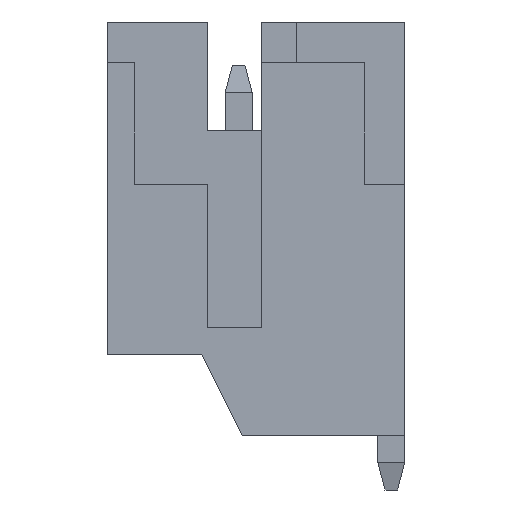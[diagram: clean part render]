
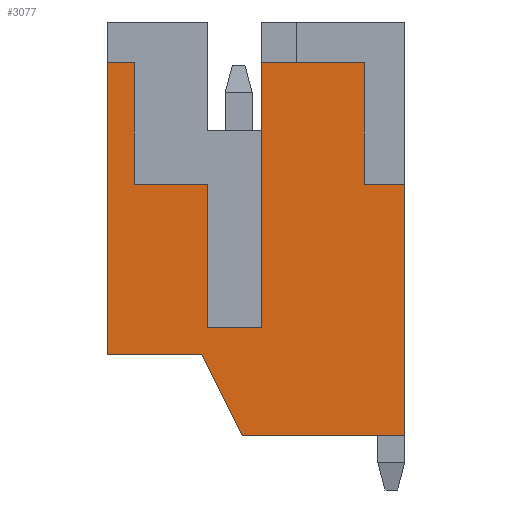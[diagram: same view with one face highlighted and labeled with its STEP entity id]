
A CAD part, left-side view. The second image highlights one B-rep face of the part: STEP entity #3077.
In plain terms, the highlighted planar face has unit normal (-1, 0, 0).
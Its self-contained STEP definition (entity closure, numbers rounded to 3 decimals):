
#189 = VECTOR ( 'NONE', #1223, 1000. ) ;
#318 = ORIENTED_EDGE ( 'NONE', *, *, #1858, .T. ) ;
#328 = EDGE_CURVE ( 'NONE', #849, #3719, #3803, .T. ) ;
#337 = VERTEX_POINT ( 'NONE', #3031 ) ;
#357 = VERTEX_POINT ( 'NONE', #2539 ) ;
#428 = ORIENTED_EDGE ( 'NONE', *, *, #328, .T. ) ;
#443 = LINE ( 'NONE', #1220, #504 ) ;
#460 = ORIENTED_EDGE ( 'NONE', *, *, #1453, .T. ) ;
#504 = VECTOR ( 'NONE', #2989, 1000. ) ;
#511 = VECTOR ( 'NONE', #5142, 1000. ) ;
#660 = AXIS2_PLACEMENT_3D ( 'NONE', #684, #3862, #2910 ) ;
#679 = CARTESIAN_POINT ( 'NONE',  ( -3., 0.58, 3.15 ) ) ;
#684 = CARTESIAN_POINT ( 'NONE',  ( -3., 0., 0. ) ) ;
#725 = DIRECTION ( 'NONE',  ( 0., 0., -1. ) ) ;
#748 = ORIENTED_EDGE ( 'NONE', *, *, #4147, .F. ) ;
#752 = CARTESIAN_POINT ( 'NONE',  ( -3., -2.32, 5.4 ) ) ;
#849 = VERTEX_POINT ( 'NONE', #5078 ) ;
#1001 = VERTEX_POINT ( 'NONE', #2383 ) ;
#1036 = CARTESIAN_POINT ( 'NONE',  ( -3., -0.42, 0.5 ) ) ;
#1052 = LINE ( 'NONE', #1036, #4838 ) ;
#1082 = CARTESIAN_POINT ( 'NONE',  ( -3., -2.32, 3.15 ) ) ;
#1083 = VERTEX_POINT ( 'NONE', #2425 ) ;
#1136 = LINE ( 'NONE', #3629, #3499 ) ;
#1220 = CARTESIAN_POINT ( 'NONE',  ( -3., -0.42, 3.15 ) ) ;
#1223 = DIRECTION ( 'NONE',  ( 0., 0., 1. ) ) ;
#1237 = DIRECTION ( 'NONE',  ( 0., -0.447, -0.894 ) ) ;
#1324 = CARTESIAN_POINT ( 'NONE',  ( -3., -3.07, 3.15 ) ) ;
#1340 = EDGE_CURVE ( 'NONE', #1083, #5493, #1136, .T. ) ;
#1410 = DIRECTION ( 'NONE',  ( 0., -1., 0. ) ) ;
#1453 = EDGE_CURVE ( 'NONE', #357, #4659, #3775, .T. ) ;
#1612 = EDGE_CURVE ( 'NONE', #5716, #2660, #2919, .T. ) ;
#1774 = LINE ( 'NONE', #1859, #5238 ) ;
#1776 = ORIENTED_EDGE ( 'NONE', *, *, #2303, .T. ) ;
#1837 = EDGE_CURVE ( 'NONE', #337, #3189, #443, .T. ) ;
#1858 = EDGE_CURVE ( 'NONE', #5353, #1001, #1920, .T. ) ;
#1859 = CARTESIAN_POINT ( 'NONE',  ( -3., -2.32, 3.15 ) ) ;
#1920 = LINE ( 'NONE', #4403, #3068 ) ;
#1964 = EDGE_CURVE ( 'NONE', #4659, #2823, #5400, .T. ) ;
#1966 = LINE ( 'NONE', #679, #2693 ) ;
#1997 = CARTESIAN_POINT ( 'NONE',  ( -3., -3.07, -1.5 ) ) ;
#2003 = DIRECTION ( 'NONE',  ( 0., 0., 1. ) ) ;
#2010 = FACE_OUTER_BOUND ( 'NONE', #4654, .T. ) ;
#2022 = CARTESIAN_POINT ( 'NONE',  ( -3., 1.93, 3.15 ) ) ;
#2059 = CARTESIAN_POINT ( 'NONE',  ( -3., -3.07, 6.15 ) ) ;
#2167 = ORIENTED_EDGE ( 'NONE', *, *, #2232, .F. ) ;
#2177 = DIRECTION ( 'NONE',  ( 0., 0., -1. ) ) ;
#2206 = ORIENTED_EDGE ( 'NONE', *, *, #3909, .F. ) ;
#2232 = EDGE_CURVE ( 'NONE', #2406, #1001, #1052, .T. ) ;
#2265 = CARTESIAN_POINT ( 'NONE',  ( -3., 2.43, 6.15 ) ) ;
#2303 = EDGE_CURVE ( 'NONE', #2823, #849, #3761, .T. ) ;
#2357 = CARTESIAN_POINT ( 'NONE',  ( -3., 2.43, 0. ) ) ;
#2383 = CARTESIAN_POINT ( 'NONE',  ( -3., -0.42, 0.5 ) ) ;
#2401 = CARTESIAN_POINT ( 'NONE',  ( -3., -2.32, 3.15 ) ) ;
#2406 = VERTEX_POINT ( 'NONE', #3804 ) ;
#2425 = CARTESIAN_POINT ( 'NONE',  ( -3., 1.93, 5.4 ) ) ;
#2490 = LINE ( 'NONE', #3067, #3404 ) ;
#2539 = CARTESIAN_POINT ( 'NONE',  ( -3., 2.43, 0. ) ) ;
#2566 = VECTOR ( 'NONE', #2915, 1000. ) ;
#2660 = VERTEX_POINT ( 'NONE', #752 ) ;
#2693 = VECTOR ( 'NONE', #725, 1000. ) ;
#2758 = DIRECTION ( 'NONE',  ( 0., 1., 0. ) ) ;
#2783 = EDGE_CURVE ( 'NONE', #2660, #5353, #2490, .T. ) ;
#2819 = VECTOR ( 'NONE', #2003, 1000. ) ;
#2823 = VERTEX_POINT ( 'NONE', #4219 ) ;
#2910 = DIRECTION ( 'NONE',  ( 0., -1., 0. ) ) ;
#2915 = DIRECTION ( 'NONE',  ( 0., -1., 0. ) ) ;
#2919 = LINE ( 'NONE', #1082, #511 ) ;
#2989 = DIRECTION ( 'NONE',  ( 0., -1., 0. ) ) ;
#3031 = CARTESIAN_POINT ( 'NONE',  ( -3., 1.93, 3.15 ) ) ;
#3042 = CARTESIAN_POINT ( 'NONE',  ( -3., -0.42, 5.4 ) ) ;
#3067 = CARTESIAN_POINT ( 'NONE',  ( -3., -3.07, 5.4 ) ) ;
#3068 = VECTOR ( 'NONE', #5706, 1000. ) ;
#3077 = ADVANCED_FACE ( 'NONE', ( #2010 ), #3414, .T. ) ;
#3189 = VERTEX_POINT ( 'NONE', #4826 ) ;
#3285 = ORIENTED_EDGE ( 'NONE', *, *, #2783, .T. ) ;
#3359 = VECTOR ( 'NONE', #5503, 1000. ) ;
#3367 = CARTESIAN_POINT ( 'NONE',  ( -3., 0.68, 0. ) ) ;
#3404 = VECTOR ( 'NONE', #2758, 1000. ) ;
#3414 = PLANE ( 'NONE',  #660 ) ;
#3499 = VECTOR ( 'NONE', #4959, 1000. ) ;
#3508 = EDGE_CURVE ( 'NONE', #5493, #357, #5245, .T. ) ;
#3526 = ORIENTED_EDGE ( 'NONE', *, *, #3508, .T. ) ;
#3540 = CARTESIAN_POINT ( 'NONE',  ( -3., -0.07, -1.5 ) ) ;
#3629 = CARTESIAN_POINT ( 'NONE',  ( -3., -3.07, 5.4 ) ) ;
#3688 = VECTOR ( 'NONE', #2177, 1000. ) ;
#3719 = VERTEX_POINT ( 'NONE', #1324 ) ;
#3761 = LINE ( 'NONE', #1997, #2566 ) ;
#3775 = LINE ( 'NONE', #2357, #3359 ) ;
#3786 = ORIENTED_EDGE ( 'NONE', *, *, #1837, .F. ) ;
#3803 = LINE ( 'NONE', #2059, #189 ) ;
#3804 = CARTESIAN_POINT ( 'NONE',  ( -3., 0.58, 0.5 ) ) ;
#3862 = DIRECTION ( 'NONE',  ( -1., 0., 0. ) ) ;
#3909 = EDGE_CURVE ( 'NONE', #5716, #3719, #1774, .T. ) ;
#4147 = EDGE_CURVE ( 'NONE', #3189, #2406, #1966, .T. ) ;
#4189 = DIRECTION ( 'NONE',  ( 0., -1., 0. ) ) ;
#4219 = CARTESIAN_POINT ( 'NONE',  ( -3., -0.07, -1.5 ) ) ;
#4275 = ORIENTED_EDGE ( 'NONE', *, *, #4676, .T. ) ;
#4403 = CARTESIAN_POINT ( 'NONE',  ( -3., -0.42, 6.15 ) ) ;
#4654 = EDGE_LOOP ( 'NONE', ( #4948, #3526, #460, #5448, #1776, #428, #2206, #5410, #3285, #318, #2167, #748, #3786, #4275 ) ) ;
#4659 = VERTEX_POINT ( 'NONE', #3367 ) ;
#4676 = EDGE_CURVE ( 'NONE', #337, #1083, #4818, .T. ) ;
#4818 = LINE ( 'NONE', #2022, #2819 ) ;
#4826 = CARTESIAN_POINT ( 'NONE',  ( -3., 0.58, 3.15 ) ) ;
#4838 = VECTOR ( 'NONE', #4189, 1000. ) ;
#4931 = CARTESIAN_POINT ( 'NONE',  ( -3., 2.43, 5.4 ) ) ;
#4948 = ORIENTED_EDGE ( 'NONE', *, *, #1340, .T. ) ;
#4959 = DIRECTION ( 'NONE',  ( 0., 1., 0. ) ) ;
#5078 = CARTESIAN_POINT ( 'NONE',  ( -3., -3.07, -1.5 ) ) ;
#5118 = VECTOR ( 'NONE', #1237, 1000. ) ;
#5142 = DIRECTION ( 'NONE',  ( 0., 0., 1. ) ) ;
#5238 = VECTOR ( 'NONE', #1410, 1000. ) ;
#5245 = LINE ( 'NONE', #2265, #3688 ) ;
#5353 = VERTEX_POINT ( 'NONE', #3042 ) ;
#5400 = LINE ( 'NONE', #3540, #5118 ) ;
#5410 = ORIENTED_EDGE ( 'NONE', *, *, #1612, .T. ) ;
#5448 = ORIENTED_EDGE ( 'NONE', *, *, #1964, .T. ) ;
#5493 = VERTEX_POINT ( 'NONE', #4931 ) ;
#5503 = DIRECTION ( 'NONE',  ( 0., -1., 0. ) ) ;
#5706 = DIRECTION ( 'NONE',  ( 0., 0., -1. ) ) ;
#5716 = VERTEX_POINT ( 'NONE', #2401 ) ;
